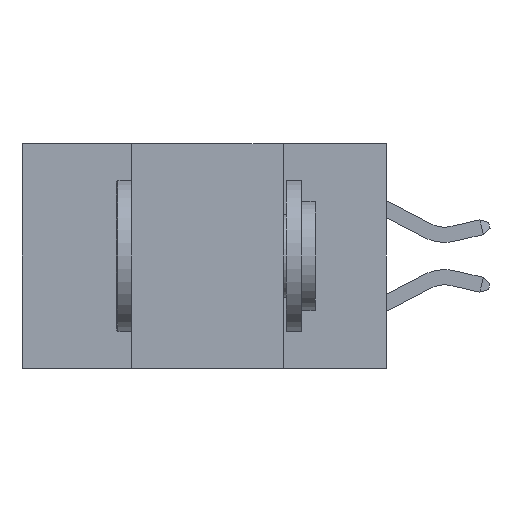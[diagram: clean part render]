
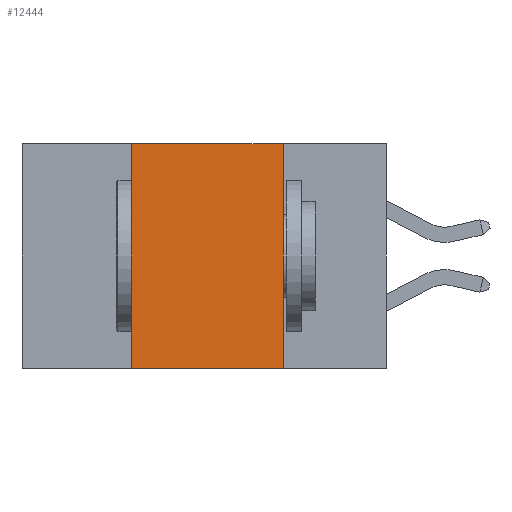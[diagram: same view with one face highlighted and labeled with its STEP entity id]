
A CAD part, left-side view. The second image highlights one B-rep face of the part: STEP entity #12444.
In plain terms, the highlighted planar face has unit normal (-1, 0, 0).
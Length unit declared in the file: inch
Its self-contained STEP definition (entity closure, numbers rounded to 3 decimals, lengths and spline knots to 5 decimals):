
#271 = ORIENTED_EDGE ( 'NONE', *, *, #9317, .T. ) ;
#337 = VERTEX_POINT ( 'NONE', #11736 ) ;
#660 = VERTEX_POINT ( 'NONE', #7509 ) ;
#1265 = LINE ( 'NONE', #1985, #10072 ) ;
#1985 = CARTESIAN_POINT ( 'NONE',  ( 0., 0.42, 0. ) ) ;
#2695 = EDGE_CURVE ( 'NONE', #20966, #660, #4297, .T. ) ;
#3777 = CARTESIAN_POINT ( 'NONE',  ( 0., 0.6, 0. ) ) ;
#3828 = CARTESIAN_POINT ( 'NONE',  ( 0., 0.6, 0. ) ) ;
#3892 = DIRECTION ( 'NONE',  ( 0., -1., 0. ) ) ;
#4297 = LINE ( 'NONE', #18479, #8408 ) ;
#4431 = ORIENTED_EDGE ( 'NONE', *, *, #8589, .F. ) ;
#5943 = LINE ( 'NONE', #3828, #14151 ) ;
#6888 = ORIENTED_EDGE ( 'NONE', *, *, #2695, .F. ) ;
#7509 = CARTESIAN_POINT ( 'NONE',  ( 0., 0.17, -0.37 ) ) ;
#8408 = VECTOR ( 'NONE', #18861, 39.37008 ) ;
#8589 = EDGE_CURVE ( 'NONE', #337, #15254, #1265, .T. ) ;
#9063 = DIRECTION ( 'NONE',  ( 1., 0., 0. ) ) ;
#9207 = CARTESIAN_POINT ( 'NONE',  ( 0., 0.42, 0. ) ) ;
#9317 = EDGE_CURVE ( 'NONE', #337, #660, #13595, .T. ) ;
#10072 = VECTOR ( 'NONE', #12446, 39.37008 ) ;
#10979 = EDGE_LOOP ( 'NONE', ( #6888, #17780, #4431, #271 ) ) ;
#11736 = CARTESIAN_POINT ( 'NONE',  ( 0., 0.42, -0.37 ) ) ;
#12444 = ADVANCED_FACE ( 'NONE', ( #17432 ), #19441, .F. ) ;
#12446 = DIRECTION ( 'NONE',  ( 0., 0., 1. ) ) ;
#12574 = CARTESIAN_POINT ( 'NONE',  ( 0., 0.6, -0.37 ) ) ;
#13016 = EDGE_CURVE ( 'NONE', #15254, #20966, #5943, .T. ) ;
#13595 = LINE ( 'NONE', #12574, #22261 ) ;
#13992 = CARTESIAN_POINT ( 'NONE',  ( 0., 0.17, 0. ) ) ;
#14151 = VECTOR ( 'NONE', #14296, 39.37008 ) ;
#14296 = DIRECTION ( 'NONE',  ( 0., -1., 0. ) ) ;
#15254 = VERTEX_POINT ( 'NONE', #9207 ) ;
#17432 = FACE_OUTER_BOUND ( 'NONE', #10979, .T. ) ;
#17780 = ORIENTED_EDGE ( 'NONE', *, *, #13016, .F. ) ;
#18479 = CARTESIAN_POINT ( 'NONE',  ( 0., 0.17, 0. ) ) ;
#18861 = DIRECTION ( 'NONE',  ( 0., 0., -1. ) ) ;
#19441 = PLANE ( 'NONE',  #20316 ) ;
#20316 = AXIS2_PLACEMENT_3D ( 'NONE', #3777, #9063, #21176 ) ;
#20966 = VERTEX_POINT ( 'NONE', #13992 ) ;
#21176 = DIRECTION ( 'NONE',  ( 0., 0., -1. ) ) ;
#22261 = VECTOR ( 'NONE', #3892, 39.37008 ) ;
